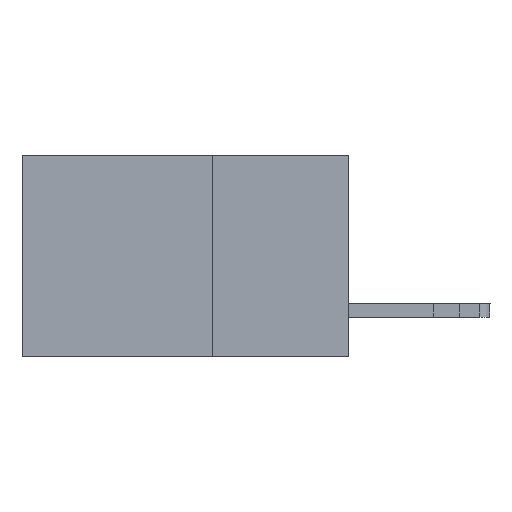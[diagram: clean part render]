
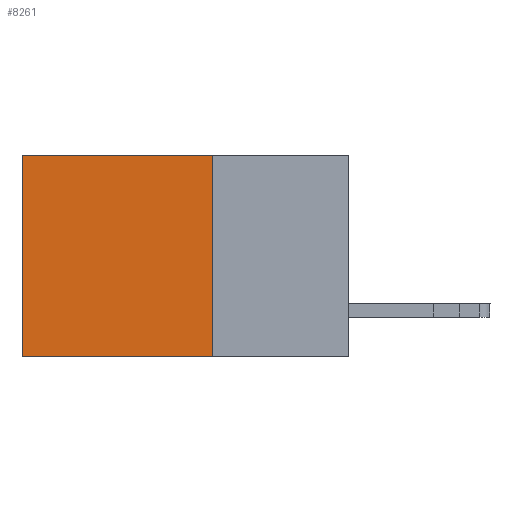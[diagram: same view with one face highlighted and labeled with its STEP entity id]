
A CAD part, left-side view. The second image highlights one B-rep face of the part: STEP entity #8261.
In plain terms, the highlighted planar face has unit normal (-1, 0, 0).
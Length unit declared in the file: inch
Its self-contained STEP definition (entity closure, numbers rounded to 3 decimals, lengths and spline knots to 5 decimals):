
#163 = VERTEX_POINT ( 'NONE', #9448 ) ;
#1493 = DIRECTION ( 'NONE',  ( 1., 0., 0. ) ) ;
#1510 = LINE ( 'NONE', #2680, #8208 ) ;
#1662 = CARTESIAN_POINT ( 'NONE',  ( 0.2615, 0.6, 0. ) ) ;
#1668 = DIRECTION ( 'NONE',  ( 0., 1., 0. ) ) ;
#1845 = AXIS2_PLACEMENT_3D ( 'NONE', #6733, #1493, #11051 ) ;
#2680 = CARTESIAN_POINT ( 'NONE',  ( 0.2615, 0.25, -0.37 ) ) ;
#2727 = LINE ( 'NONE', #12809, #5360 ) ;
#3025 = DIRECTION ( 'NONE',  ( 0., 1., 0. ) ) ;
#3207 = EDGE_CURVE ( 'NONE', #4888, #11002, #2727, .T. ) ;
#3244 = VERTEX_POINT ( 'NONE', #1662 ) ;
#3908 = CARTESIAN_POINT ( 'NONE',  ( 0.2615, 0.25, 0. ) ) ;
#4095 = EDGE_CURVE ( 'NONE', #4888, #3244, #4367, .T. ) ;
#4123 = ORIENTED_EDGE ( 'NONE', *, *, #8250, .F. ) ;
#4367 = LINE ( 'NONE', #3908, #10379 ) ;
#4425 = CARTESIAN_POINT ( 'NONE',  ( 0.2615, 0.6, -0.37 ) ) ;
#4888 = VERTEX_POINT ( 'NONE', #10550 ) ;
#5091 = ORIENTED_EDGE ( 'NONE', *, *, #4095, .T. ) ;
#5360 = VECTOR ( 'NONE', #11842, 39.37008 ) ;
#5441 = FACE_OUTER_BOUND ( 'NONE', #9711, .T. ) ;
#5451 = VECTOR ( 'NONE', #5466, 39.37008 ) ;
#5466 = DIRECTION ( 'NONE',  ( 0., 0., -1. ) ) ;
#5832 = EDGE_CURVE ( 'NONE', #3244, #163, #6247, .T. ) ;
#6247 = LINE ( 'NONE', #4425, #5451 ) ;
#6733 = CARTESIAN_POINT ( 'NONE',  ( 0.2615, 0.25, -0.37 ) ) ;
#8208 = VECTOR ( 'NONE', #1668, 39.37008 ) ;
#8250 = EDGE_CURVE ( 'NONE', #11002, #163, #1510, .T. ) ;
#8261 = ADVANCED_FACE ( 'NONE', ( #5441 ), #13041, .F. ) ;
#9448 = CARTESIAN_POINT ( 'NONE',  ( 0.2615, 0.6, -0.37 ) ) ;
#9711 = EDGE_LOOP ( 'NONE', ( #10511, #4123, #13227, #5091 ) ) ;
#10379 = VECTOR ( 'NONE', #3025, 39.37008 ) ;
#10511 = ORIENTED_EDGE ( 'NONE', *, *, #5832, .T. ) ;
#10550 = CARTESIAN_POINT ( 'NONE',  ( 0.2615, 0.25, 0. ) ) ;
#11002 = VERTEX_POINT ( 'NONE', #13061 ) ;
#11051 = DIRECTION ( 'NONE',  ( 0., 0., -1. ) ) ;
#11842 = DIRECTION ( 'NONE',  ( 0., 0., -1. ) ) ;
#12809 = CARTESIAN_POINT ( 'NONE',  ( 0.2615, 0.25, -0.37 ) ) ;
#13041 = PLANE ( 'NONE',  #1845 ) ;
#13061 = CARTESIAN_POINT ( 'NONE',  ( 0.2615, 0.25, -0.37 ) ) ;
#13227 = ORIENTED_EDGE ( 'NONE', *, *, #3207, .F. ) ;
